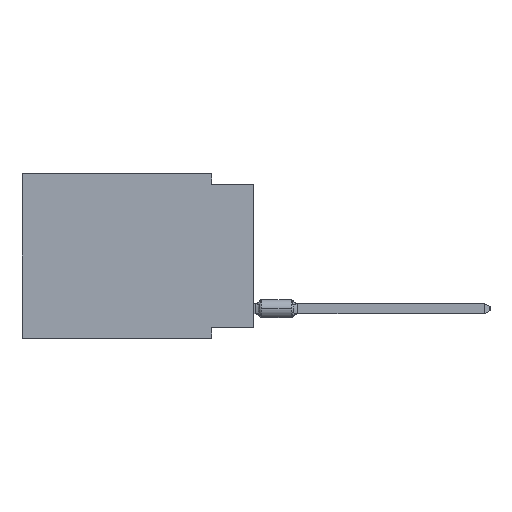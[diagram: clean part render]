
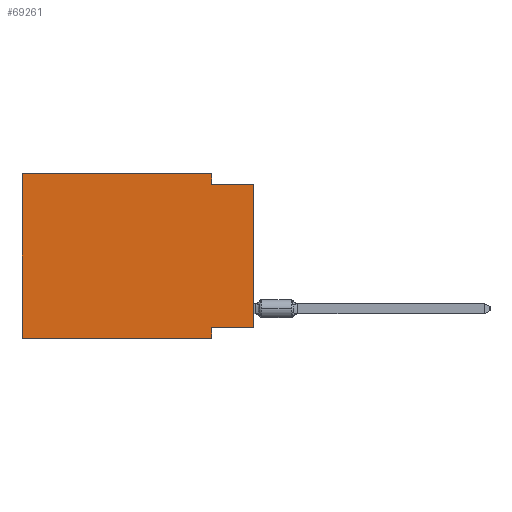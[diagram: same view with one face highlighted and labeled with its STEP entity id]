
A CAD part, left-side view. The second image highlights one B-rep face of the part: STEP entity #69261.
In plain terms, the highlighted planar face has unit normal (-1, 0, 0).
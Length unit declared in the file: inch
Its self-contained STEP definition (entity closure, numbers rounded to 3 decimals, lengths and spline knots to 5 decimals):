
#111 = CARTESIAN_POINT ( 'NONE',  ( 0., 0., 0. ) ) ;
#1458 = FACE_OUTER_BOUND ( 'NONE', #65159, .T. ) ;
#3052 = VECTOR ( 'NONE', #18037, 39.37008 ) ;
#5884 = VECTOR ( 'NONE', #27432, 39.37008 ) ;
#6058 = VECTOR ( 'NONE', #33141, 39.37008 ) ;
#6082 = VECTOR ( 'NONE', #8715, 39.37008 ) ;
#6143 = CARTESIAN_POINT ( 'NONE',  ( 0., 0., -0.025 ) ) ;
#6643 = DIRECTION ( 'NONE',  ( 1., 0., 0. ) ) ;
#6987 = CARTESIAN_POINT ( 'NONE',  ( 0., 0.55, 0. ) ) ;
#7261 = ORIENTED_EDGE ( 'NONE', *, *, #39884, .F. ) ;
#7542 = VERTEX_POINT ( 'NONE', #18176 ) ;
#8715 = DIRECTION ( 'NONE',  ( 0., -1., 0. ) ) ;
#9503 = EDGE_CURVE ( 'NONE', #59005, #60885, #33875, .T. ) ;
#9987 = ORIENTED_EDGE ( 'NONE', *, *, #48874, .F. ) ;
#10399 = CARTESIAN_POINT ( 'NONE',  ( 0., 0., -0.365 ) ) ;
#10441 = LINE ( 'NONE', #111, #5884 ) ;
#10632 = CARTESIAN_POINT ( 'NONE',  ( 0., 0., -0.365 ) ) ;
#10639 = CARTESIAN_POINT ( 'NONE',  ( 0., 0.55, 0. ) ) ;
#12862 = DIRECTION ( 'NONE',  ( 0., 0., -1. ) ) ;
#16387 = EDGE_CURVE ( 'NONE', #59005, #7542, #44242, .T. ) ;
#16524 = CARTESIAN_POINT ( 'NONE',  ( 0., 0.55, -0.39 ) ) ;
#18037 = DIRECTION ( 'NONE',  ( 0., 0., -1. ) ) ;
#18176 = CARTESIAN_POINT ( 'NONE',  ( 0., 0.1, -0.39 ) ) ;
#18479 = ORIENTED_EDGE ( 'NONE', *, *, #57353, .F. ) ;
#20558 = LINE ( 'NONE', #26457, #27187 ) ;
#21924 = ORIENTED_EDGE ( 'NONE', *, *, #37143, .F. ) ;
#23232 = PLANE ( 'NONE',  #33817 ) ;
#25004 = DIRECTION ( 'NONE',  ( 0., 0., -1. ) ) ;
#26457 = CARTESIAN_POINT ( 'NONE',  ( 0., 0.1, -0.39 ) ) ;
#27187 = VECTOR ( 'NONE', #25004, 39.37008 ) ;
#27432 = DIRECTION ( 'NONE',  ( 0., 0., 1. ) ) ;
#32078 = VERTEX_POINT ( 'NONE', #10399 ) ;
#32406 = LINE ( 'NONE', #10632, #33463 ) ;
#33141 = DIRECTION ( 'NONE',  ( 0., 0., 1. ) ) ;
#33463 = VECTOR ( 'NONE', #54973, 39.37008 ) ;
#33817 = AXIS2_PLACEMENT_3D ( 'NONE', #6987, #6643, #12862 ) ;
#33875 = LINE ( 'NONE', #10639, #6058 ) ;
#36772 = LINE ( 'NONE', #59331, #6082 ) ;
#37143 = EDGE_CURVE ( 'NONE', #43653, #7542, #20558, .T. ) ;
#37614 = CARTESIAN_POINT ( 'NONE',  ( 0., 0.55, 0. ) ) ;
#38540 = VERTEX_POINT ( 'NONE', #56375 ) ;
#39021 = LINE ( 'NONE', #50485, #50604 ) ;
#39076 = DIRECTION ( 'NONE',  ( 0., -1., 0. ) ) ;
#39884 = EDGE_CURVE ( 'NONE', #40585, #50626, #39021, .T. ) ;
#40585 = VERTEX_POINT ( 'NONE', #54016 ) ;
#42105 = EDGE_CURVE ( 'NONE', #32078, #50626, #10441, .T. ) ;
#43653 = VERTEX_POINT ( 'NONE', #54373 ) ;
#44242 = LINE ( 'NONE', #16524, #72289 ) ;
#45853 = ORIENTED_EDGE ( 'NONE', *, *, #51452, .F. ) ;
#46111 = LINE ( 'NONE', #50956, #3052 ) ;
#48874 = EDGE_CURVE ( 'NONE', #32078, #43653, #32406, .T. ) ;
#50485 = CARTESIAN_POINT ( 'NONE',  ( 0., 0., -0.025 ) ) ;
#50604 = VECTOR ( 'NONE', #61570, 39.37008 ) ;
#50626 = VERTEX_POINT ( 'NONE', #6143 ) ;
#50956 = CARTESIAN_POINT ( 'NONE',  ( 0., 0.1, 0. ) ) ;
#51452 = EDGE_CURVE ( 'NONE', #38540, #40585, #46111, .T. ) ;
#51582 = ORIENTED_EDGE ( 'NONE', *, *, #16387, .T. ) ;
#54016 = CARTESIAN_POINT ( 'NONE',  ( 0., 0.1, -0.025 ) ) ;
#54373 = CARTESIAN_POINT ( 'NONE',  ( 0., 0.1, -0.365 ) ) ;
#54973 = DIRECTION ( 'NONE',  ( 0., 1., 0. ) ) ;
#55477 = CARTESIAN_POINT ( 'NONE',  ( 0., 0.55, -0.39 ) ) ;
#56375 = CARTESIAN_POINT ( 'NONE',  ( 0., 0.1, 0. ) ) ;
#57353 = EDGE_CURVE ( 'NONE', #60885, #38540, #36772, .T. ) ;
#59005 = VERTEX_POINT ( 'NONE', #55477 ) ;
#59331 = CARTESIAN_POINT ( 'NONE',  ( 0., 0.55, 0. ) ) ;
#59646 = ORIENTED_EDGE ( 'NONE', *, *, #42105, .T. ) ;
#60885 = VERTEX_POINT ( 'NONE', #37614 ) ;
#61570 = DIRECTION ( 'NONE',  ( 0., -1., 0. ) ) ;
#65159 = EDGE_LOOP ( 'NONE', ( #59646, #7261, #45853, #18479, #71594, #51582, #21924, #9987 ) ) ;
#69261 = ADVANCED_FACE ( 'NONE', ( #1458 ), #23232, .F. ) ;
#71594 = ORIENTED_EDGE ( 'NONE', *, *, #9503, .F. ) ;
#72289 = VECTOR ( 'NONE', #39076, 39.37008 ) ;
